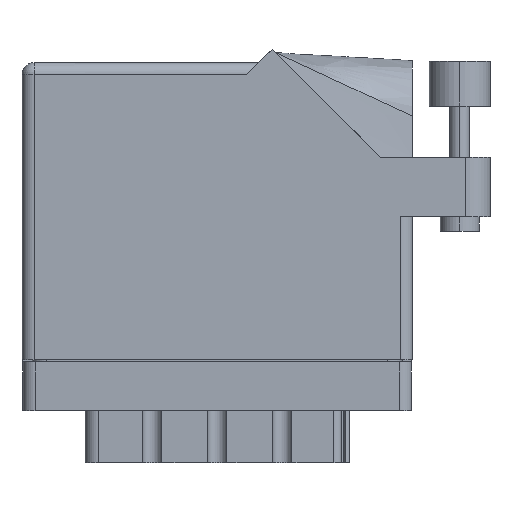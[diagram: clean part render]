
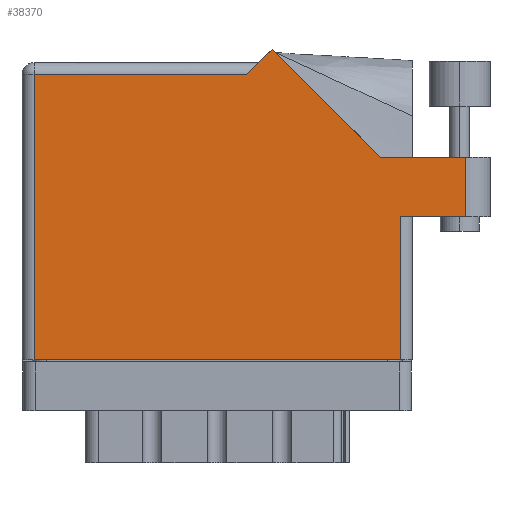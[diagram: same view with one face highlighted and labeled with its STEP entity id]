
A CAD part, front view. The second image highlights one B-rep face of the part: STEP entity #38370.
In plain terms, the highlighted face is planar.
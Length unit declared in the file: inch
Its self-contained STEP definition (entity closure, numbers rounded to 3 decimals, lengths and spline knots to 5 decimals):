
#708 = ORIENTED_EDGE ( 'NONE', *, *, #11498, .T. ) ;
#725 = EDGE_CURVE ( 'NONE', #40067, #24897, #811, .T. ) ;
#811 = LINE ( 'NONE', #28589, #5819 ) ;
#1484 = PLANE ( 'NONE',  #11449 ) ;
#1668 = CARTESIAN_POINT ( 'NONE',  ( 2.285, 1.044, 0. ) ) ;
#1773 = FACE_OUTER_BOUND ( 'NONE', #33170, .T. ) ;
#3100 = ORIENTED_EDGE ( 'NONE', *, *, #29132, .T. ) ;
#3283 = ORIENTED_EDGE ( 'NONE', *, *, #725, .T. ) ;
#3505 = ORIENTED_EDGE ( 'NONE', *, *, #27177, .T. ) ;
#3595 = LINE ( 'NONE', #24602, #20980 ) ;
#3930 = VECTOR ( 'NONE', #15442, 39.37008 ) ;
#4700 = DIRECTION ( 'NONE',  ( 0., 0., -1. ) ) ;
#5547 = DIRECTION ( 'NONE',  ( 0., -1., 0. ) ) ;
#5819 = VECTOR ( 'NONE', #31745, 39.37008 ) ;
#6426 = LINE ( 'NONE', #31949, #3930 ) ;
#6507 = ORIENTED_EDGE ( 'NONE', *, *, #26964, .T. ) ;
#7161 = VERTEX_POINT ( 'NONE', #24165 ) ;
#9208 = EDGE_CURVE ( 'NONE', #26379, #32418, #27569, .T. ) ;
#9418 = CARTESIAN_POINT ( 'NONE',  ( 1.155, 1.468, 0. ) ) ;
#9715 = VERTEX_POINT ( 'NONE', #9418 ) ;
#10632 = LINE ( 'NONE', #17814, #31954 ) ;
#10936 = CARTESIAN_POINT ( 'NONE',  ( 0., 0., 0. ) ) ;
#11449 = AXIS2_PLACEMENT_3D ( 'NONE', #33426, #4700, #36225 ) ;
#11498 = EDGE_CURVE ( 'NONE', #31559, #31045, #29912, .T. ) ;
#13032 = VECTOR ( 'NONE', #26614, 39.37008 ) ;
#13281 = CARTESIAN_POINT ( 'NONE',  ( 0.062, 1.468, 0. ) ) ;
#15442 = DIRECTION ( 'NONE',  ( -1., 0., 0. ) ) ;
#15821 = EDGE_CURVE ( 'NONE', #7161, #26379, #6426, .T. ) ;
#15878 = DIRECTION ( 'NONE',  ( -1., 0., 0. ) ) ;
#17649 = CARTESIAN_POINT ( 'NONE',  ( 1.948, 0., 0. ) ) ;
#17814 = CARTESIAN_POINT ( 'NONE',  ( 1.948, 0.737, 0. ) ) ;
#19446 = DIRECTION ( 'NONE',  ( -0.707, 0.707, 0. ) ) ;
#19814 = CARTESIAN_POINT ( 'NONE',  ( 1.84442, 1.044, 0. ) ) ;
#20980 = VECTOR ( 'NONE', #5547, 39.37008 ) ;
#21098 = VECTOR ( 'NONE', #19446, 39.37008 ) ;
#21233 = VECTOR ( 'NONE', #26152, 39.37008 ) ;
#22911 = EDGE_CURVE ( 'NONE', #31045, #40067, #10632, .T. ) ;
#23247 = CARTESIAN_POINT ( 'NONE',  ( 2.285, 0.737, 0. ) ) ;
#23408 = EDGE_CURVE ( 'NONE', #38792, #31559, #3595, .T. ) ;
#23792 = CARTESIAN_POINT ( 'NONE',  ( 0.062, 0., 0. ) ) ;
#24165 = CARTESIAN_POINT ( 'NONE',  ( 2.285, 1.044, 0. ) ) ;
#24602 = CARTESIAN_POINT ( 'NONE',  ( 0.062, 0., 0. ) ) ;
#24870 = CARTESIAN_POINT ( 'NONE',  ( 1.28771, 1.60071, 0. ) ) ;
#24897 = VERTEX_POINT ( 'NONE', #23247 ) ;
#26152 = DIRECTION ( 'NONE',  ( -0.707, -0.707, 0. ) ) ;
#26379 = VERTEX_POINT ( 'NONE', #19814 ) ;
#26400 = ORIENTED_EDGE ( 'NONE', *, *, #22911, .T. ) ;
#26614 = DIRECTION ( 'NONE',  ( 1., 0., 0. ) ) ;
#26964 = EDGE_CURVE ( 'NONE', #9715, #38792, #29207, .T. ) ;
#27177 = EDGE_CURVE ( 'NONE', #32418, #9715, #40138, .T. ) ;
#27569 = LINE ( 'NONE', #28903, #21098 ) ;
#28589 = CARTESIAN_POINT ( 'NONE',  ( 2.01, 0.737, 0. ) ) ;
#28770 = ORIENTED_EDGE ( 'NONE', *, *, #15821, .T. ) ;
#28811 = CARTESIAN_POINT ( 'NONE',  ( 0., 1.468, 0. ) ) ;
#28903 = CARTESIAN_POINT ( 'NONE',  ( 1.84442, 1.044, 0. ) ) ;
#29132 = EDGE_CURVE ( 'NONE', #24897, #7161, #41171, .T. ) ;
#29207 = LINE ( 'NONE', #28811, #39657 ) ;
#29912 = LINE ( 'NONE', #10936, #13032 ) ;
#31045 = VERTEX_POINT ( 'NONE', #17649 ) ;
#31559 = VERTEX_POINT ( 'NONE', #23792 ) ;
#31745 = DIRECTION ( 'NONE',  ( 1., 0., 0. ) ) ;
#31949 = CARTESIAN_POINT ( 'NONE',  ( 2.41, 1.044, 0. ) ) ;
#31954 = VECTOR ( 'NONE', #36992, 39.37008 ) ;
#32418 = VERTEX_POINT ( 'NONE', #24870 ) ;
#33170 = EDGE_LOOP ( 'NONE', ( #3283, #3100, #28770, #41149, #3505, #6507, #40520, #708, #26400 ) ) ;
#33426 = CARTESIAN_POINT ( 'NONE',  ( 0., 1.53, 0. ) ) ;
#36225 = DIRECTION ( 'NONE',  ( -1., 0., 0. ) ) ;
#36992 = DIRECTION ( 'NONE',  ( 0., 1., 0. ) ) ;
#37314 = CARTESIAN_POINT ( 'NONE',  ( 1.948, 0.737, 0. ) ) ;
#38370 = ADVANCED_FACE ( 'NONE', ( #1773 ), #1484, .F. ) ;
#38792 = VERTEX_POINT ( 'NONE', #13281 ) ;
#38804 = CARTESIAN_POINT ( 'NONE',  ( 1.217, 1.53, 0. ) ) ;
#39657 = VECTOR ( 'NONE', #15878, 39.37008 ) ;
#40067 = VERTEX_POINT ( 'NONE', #37314 ) ;
#40138 = LINE ( 'NONE', #38804, #21233 ) ;
#40294 = DIRECTION ( 'NONE',  ( 0., 1., 0. ) ) ;
#40520 = ORIENTED_EDGE ( 'NONE', *, *, #23408, .T. ) ;
#40650 = VECTOR ( 'NONE', #40294, 39.37008 ) ;
#41149 = ORIENTED_EDGE ( 'NONE', *, *, #9208, .T. ) ;
#41171 = LINE ( 'NONE', #1668, #40650 ) ;
